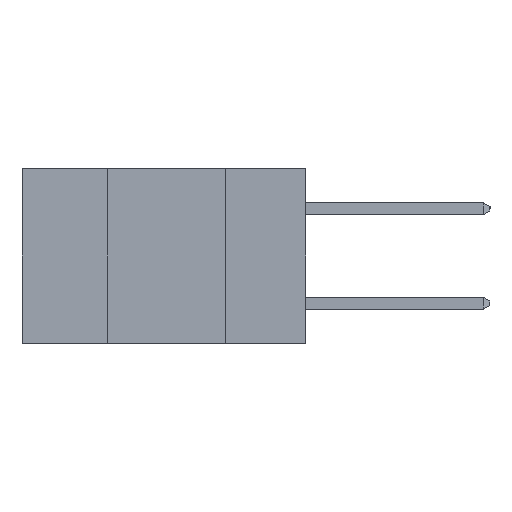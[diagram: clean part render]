
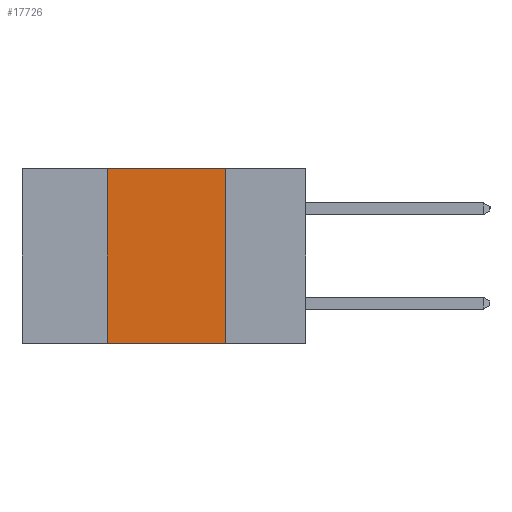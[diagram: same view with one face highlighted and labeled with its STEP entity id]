
A CAD part, left-side view. The second image highlights one B-rep face of the part: STEP entity #17726.
In plain terms, the highlighted planar face has unit normal (-1, 0, 0).
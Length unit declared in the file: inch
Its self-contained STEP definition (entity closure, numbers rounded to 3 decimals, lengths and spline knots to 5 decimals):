
#944 = ORIENTED_EDGE ( 'NONE', *, *, #20235, .F. ) ;
#2359 = VECTOR ( 'NONE', #5885, 39.37008 ) ;
#2368 = CARTESIAN_POINT ( 'NONE',  ( 0., 0.17, -0.37 ) ) ;
#2491 = VECTOR ( 'NONE', #22005, 39.37008 ) ;
#3972 = ORIENTED_EDGE ( 'NONE', *, *, #6411, .T. ) ;
#4009 = LINE ( 'NONE', #19701, #18572 ) ;
#4514 = CARTESIAN_POINT ( 'NONE',  ( 0., 0.17, 0. ) ) ;
#4905 = EDGE_LOOP ( 'NONE', ( #8064, #944, #9071, #3972 ) ) ;
#5326 = VERTEX_POINT ( 'NONE', #24833 ) ;
#5885 = DIRECTION ( 'NONE',  ( 0., -1., 0. ) ) ;
#6411 = EDGE_CURVE ( 'NONE', #19036, #8695, #23488, .T. ) ;
#6580 = DIRECTION ( 'NONE',  ( 1., 0., 0. ) ) ;
#8064 = ORIENTED_EDGE ( 'NONE', *, *, #17740, .F. ) ;
#8695 = VERTEX_POINT ( 'NONE', #12597 ) ;
#9071 = ORIENTED_EDGE ( 'NONE', *, *, #12722, .F. ) ;
#12027 = CARTESIAN_POINT ( 'NONE',  ( 0., 0.6, 0. ) ) ;
#12394 = CARTESIAN_POINT ( 'NONE',  ( 0., 0.42, -0.37 ) ) ;
#12597 = CARTESIAN_POINT ( 'NONE',  ( 0., 0.17, -0.37 ) ) ;
#12722 = EDGE_CURVE ( 'NONE', #19036, #5326, #4009, .T. ) ;
#14580 = LINE ( 'NONE', #2368, #2491 ) ;
#16379 = PLANE ( 'NONE',  #22979 ) ;
#16504 = FACE_OUTER_BOUND ( 'NONE', #4905, .T. ) ;
#17726 = ADVANCED_FACE ( 'NONE', ( #16504 ), #16379, .F. ) ;
#17740 = EDGE_CURVE ( 'NONE', #24663, #8695, #14580, .T. ) ;
#17816 = DIRECTION ( 'NONE',  ( 0., -1., 0. ) ) ;
#18572 = VECTOR ( 'NONE', #23532, 39.37008 ) ;
#19036 = VERTEX_POINT ( 'NONE', #12394 ) ;
#19399 = VECTOR ( 'NONE', #17816, 39.37008 ) ;
#19701 = CARTESIAN_POINT ( 'NONE',  ( 0., 0.42, -0.37 ) ) ;
#19849 = LINE ( 'NONE', #12027, #19399 ) ;
#20235 = EDGE_CURVE ( 'NONE', #5326, #24663, #19849, .T. ) ;
#21680 = CARTESIAN_POINT ( 'NONE',  ( 0., 0.6, -0.37 ) ) ;
#22005 = DIRECTION ( 'NONE',  ( 0., 0., -1. ) ) ;
#22252 = DIRECTION ( 'NONE',  ( 0., 0., -1. ) ) ;
#22979 = AXIS2_PLACEMENT_3D ( 'NONE', #24176, #6580, #22252 ) ;
#23488 = LINE ( 'NONE', #21680, #2359 ) ;
#23532 = DIRECTION ( 'NONE',  ( 0., 0., 1. ) ) ;
#24176 = CARTESIAN_POINT ( 'NONE',  ( 0., 0.6, 0. ) ) ;
#24663 = VERTEX_POINT ( 'NONE', #4514 ) ;
#24833 = CARTESIAN_POINT ( 'NONE',  ( 0., 0.42, 0. ) ) ;
